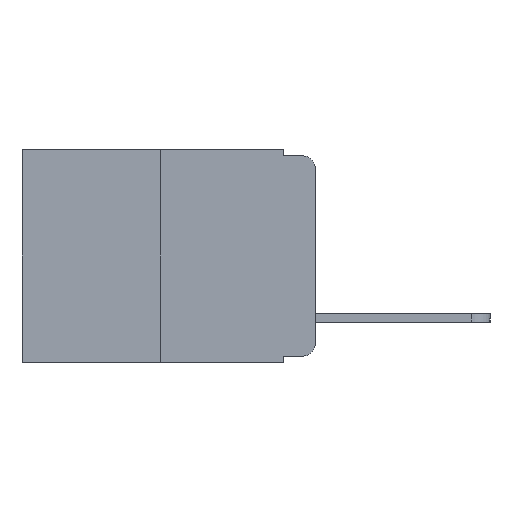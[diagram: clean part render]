
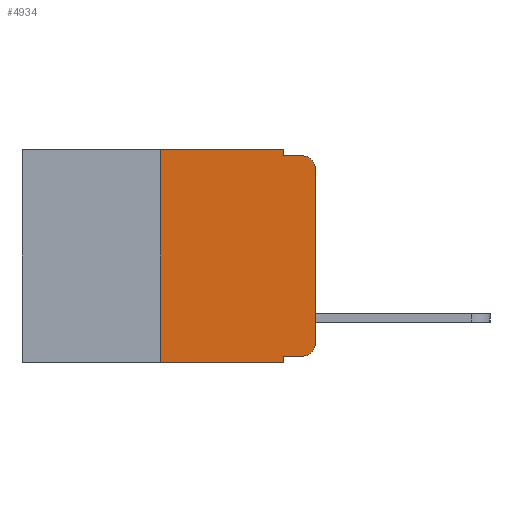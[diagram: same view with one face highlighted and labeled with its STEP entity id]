
A CAD part, left-side view. The second image highlights one B-rep face of the part: STEP entity #4934.
In plain terms, the highlighted planar face has unit normal (-1, 0, 0).
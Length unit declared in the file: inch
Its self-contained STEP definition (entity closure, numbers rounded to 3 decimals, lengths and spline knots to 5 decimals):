
#126 = CARTESIAN_POINT ( 'NONE',  ( 0., 0.25, 0. ) ) ;
#197 = ORIENTED_EDGE ( 'NONE', *, *, #8803, .F. ) ;
#257 = CARTESIAN_POINT ( 'NONE',  ( 0., 0.051, 0. ) ) ;
#372 = VERTEX_POINT ( 'NONE', #9406 ) ;
#374 = ORIENTED_EDGE ( 'NONE', *, *, #2721, .T. ) ;
#671 = DIRECTION ( 'NONE',  ( 0., 0., -1. ) ) ;
#693 = VERTEX_POINT ( 'NONE', #6505 ) ;
#1037 = VERTEX_POINT ( 'NONE', #126 ) ;
#1128 = CARTESIAN_POINT ( 'NONE',  ( 0., 0.051, -0.01 ) ) ;
#1270 = VECTOR ( 'NONE', #4734, 39.37008 ) ;
#1319 = AXIS2_PLACEMENT_3D ( 'NONE', #8335, #8289, #8277 ) ;
#1445 = EDGE_CURVE ( 'NONE', #3691, #1601, #9091, .T. ) ;
#1552 = VERTEX_POINT ( 'NONE', #8115 ) ;
#1596 = CARTESIAN_POINT ( 'NONE',  ( 0., 0.473, 0. ) ) ;
#1601 = VERTEX_POINT ( 'NONE', #3684 ) ;
#1615 = CIRCLE ( 'NONE', #7098, 0.02 ) ;
#2120 = ORIENTED_EDGE ( 'NONE', *, *, #10368, .F. ) ;
#2141 = ORIENTED_EDGE ( 'NONE', *, *, #3899, .T. ) ;
#2255 = DIRECTION ( 'NONE',  ( 0., 0., -1. ) ) ;
#2420 = CARTESIAN_POINT ( 'NONE',  ( 0., 0.051, -0.333 ) ) ;
#2534 = CARTESIAN_POINT ( 'NONE',  ( 0., 0.051, 0. ) ) ;
#2561 = ORIENTED_EDGE ( 'NONE', *, *, #1445, .T. ) ;
#2721 = EDGE_CURVE ( 'NONE', #1552, #693, #1615, .T. ) ;
#2922 = CARTESIAN_POINT ( 'NONE',  ( 0., 0.473, -0.343 ) ) ;
#2963 = CARTESIAN_POINT ( 'NONE',  ( 0., 0.051, -0.333 ) ) ;
#3066 = CARTESIAN_POINT ( 'NONE',  ( 0., 0.25, 0. ) ) ;
#3103 = EDGE_CURVE ( 'NONE', #372, #1601, #6956, .T. ) ;
#3117 = ORIENTED_EDGE ( 'NONE', *, *, #3103, .F. ) ;
#3357 = DIRECTION ( 'NONE',  ( 0., -1., 0. ) ) ;
#3544 = ORIENTED_EDGE ( 'NONE', *, *, #11274, .T. ) ;
#3606 = VERTEX_POINT ( 'NONE', #2963 ) ;
#3684 = CARTESIAN_POINT ( 'NONE',  ( 0., 0.02, -0.01 ) ) ;
#3691 = VERTEX_POINT ( 'NONE', #7065 ) ;
#3737 = VECTOR ( 'NONE', #3357, 39.37008 ) ;
#3899 = EDGE_CURVE ( 'NONE', #693, #3691, #11158, .T. ) ;
#3930 = ORIENTED_EDGE ( 'NONE', *, *, #7709, .F. ) ;
#3953 = DIRECTION ( 'NONE',  ( 0., 0., 1. ) ) ;
#3962 = CARTESIAN_POINT ( 'NONE',  ( 0., 0.051, -0.343 ) ) ;
#4111 = ORIENTED_EDGE ( 'NONE', *, *, #9871, .F. ) ;
#4177 = VECTOR ( 'NONE', #10539, 39.37008 ) ;
#4460 = LINE ( 'NONE', #9742, #4177 ) ;
#4608 = VECTOR ( 'NONE', #9432, 39.37008 ) ;
#4734 = DIRECTION ( 'NONE',  ( 0., -1., 0. ) ) ;
#4934 = ADVANCED_FACE ( 'NONE', ( #5831 ), #4970, .F. ) ;
#4939 = CARTESIAN_POINT ( 'NONE',  ( 0., 0.25, -0.343 ) ) ;
#4970 = PLANE ( 'NONE',  #5339 ) ;
#5196 = LINE ( 'NONE', #3066, #9440 ) ;
#5339 = AXIS2_PLACEMENT_3D ( 'NONE', #5850, #7611, #2255 ) ;
#5433 = VECTOR ( 'NONE', #6988, 39.37008 ) ;
#5645 = VECTOR ( 'NONE', #10751, 39.37008 ) ;
#5831 = FACE_OUTER_BOUND ( 'NONE', #10659, .T. ) ;
#5850 = CARTESIAN_POINT ( 'NONE',  ( 0., 0.473, 0. ) ) ;
#5923 = LINE ( 'NONE', #257, #5645 ) ;
#6505 = CARTESIAN_POINT ( 'NONE',  ( 0., 0., -0.313 ) ) ;
#6752 = VERTEX_POINT ( 'NONE', #4939 ) ;
#6956 = LINE ( 'NONE', #1128, #4608 ) ;
#6988 = DIRECTION ( 'NONE',  ( 0., -1., 0. ) ) ;
#6990 = VERTEX_POINT ( 'NONE', #2534 ) ;
#7065 = CARTESIAN_POINT ( 'NONE',  ( 0., 0., -0.03 ) ) ;
#7098 = AXIS2_PLACEMENT_3D ( 'NONE', #7289, #7287, #671 ) ;
#7287 = DIRECTION ( 'NONE',  ( -1., 0., 0. ) ) ;
#7289 = CARTESIAN_POINT ( 'NONE',  ( 0., 0.02, -0.313 ) ) ;
#7304 = ORIENTED_EDGE ( 'NONE', *, *, #10940, .T. ) ;
#7496 = LINE ( 'NONE', #1596, #5433 ) ;
#7550 = DIRECTION ( 'NONE',  ( 0., 0., 1. ) ) ;
#7611 = DIRECTION ( 'NONE',  ( 1., 0., 0. ) ) ;
#7709 = EDGE_CURVE ( 'NONE', #6990, #372, #5923, .T. ) ;
#8115 = CARTESIAN_POINT ( 'NONE',  ( 0., 0.02, -0.333 ) ) ;
#8277 = DIRECTION ( 'NONE',  ( 0., 0., -1. ) ) ;
#8289 = DIRECTION ( 'NONE',  ( -1., 0., 0. ) ) ;
#8335 = CARTESIAN_POINT ( 'NONE',  ( 0., 0.02, -0.03 ) ) ;
#8344 = VERTEX_POINT ( 'NONE', #3962 ) ;
#8406 = LINE ( 'NONE', #2922, #1270 ) ;
#8803 = EDGE_CURVE ( 'NONE', #6752, #1037, #5196, .T. ) ;
#9091 = CIRCLE ( 'NONE', #1319, 0.02 ) ;
#9406 = CARTESIAN_POINT ( 'NONE',  ( 0., 0.051, -0.01 ) ) ;
#9432 = DIRECTION ( 'NONE',  ( 0., -1., 0. ) ) ;
#9436 = CARTESIAN_POINT ( 'NONE',  ( 0., 0., 0. ) ) ;
#9440 = VECTOR ( 'NONE', #3953, 39.37008 ) ;
#9742 = CARTESIAN_POINT ( 'NONE',  ( 0., 0.051, 0. ) ) ;
#9871 = EDGE_CURVE ( 'NONE', #3606, #8344, #4460, .T. ) ;
#10368 = EDGE_CURVE ( 'NONE', #1037, #6990, #7496, .T. ) ;
#10539 = DIRECTION ( 'NONE',  ( 0., 0., -1. ) ) ;
#10639 = VECTOR ( 'NONE', #7550, 39.37008 ) ;
#10659 = EDGE_LOOP ( 'NONE', ( #2141, #2561, #3117, #3930, #2120, #197, #3544, #4111, #7304, #374 ) ) ;
#10751 = DIRECTION ( 'NONE',  ( 0., 0., -1. ) ) ;
#10765 = LINE ( 'NONE', #2420, #3737 ) ;
#10940 = EDGE_CURVE ( 'NONE', #3606, #1552, #10765, .T. ) ;
#11158 = LINE ( 'NONE', #9436, #10639 ) ;
#11274 = EDGE_CURVE ( 'NONE', #6752, #8344, #8406, .T. ) ;
